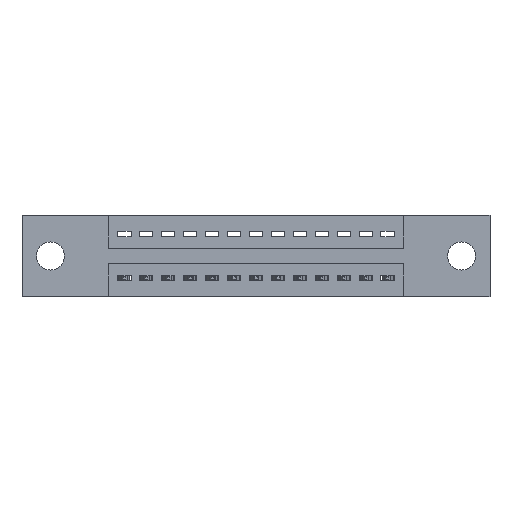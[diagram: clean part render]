
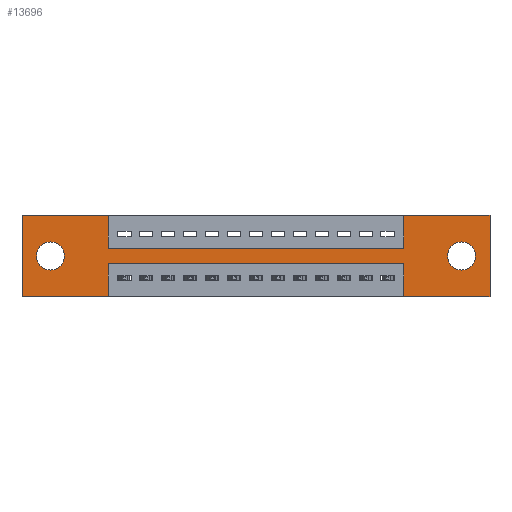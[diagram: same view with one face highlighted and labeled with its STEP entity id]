
A CAD part, front view. The second image highlights one B-rep face of the part: STEP entity #13696.
In plain terms, the highlighted planar face has unit normal (0, -1, 0).
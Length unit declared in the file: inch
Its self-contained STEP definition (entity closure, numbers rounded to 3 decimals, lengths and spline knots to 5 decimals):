
#42 = LINE ( 'NONE', #5248, #10947 ) ;
#121 = EDGE_CURVE ( 'NONE', #9580, #6579, #426, .T. ) ;
#156 = ORIENTED_EDGE ( 'NONE', *, *, #5847, .F. ) ;
#426 = LINE ( 'NONE', #842, #11322 ) ;
#506 = CIRCLE ( 'NONE', #10358, 0.064 ) ;
#594 = EDGE_CURVE ( 'NONE', #8897, #5852, #12812, .T. ) ;
#663 = EDGE_LOOP ( 'NONE', ( #5602, #11993 ) ) ;
#673 = DIRECTION ( 'NONE',  ( 1., 0., 0. ) ) ;
#752 = CARTESIAN_POINT ( 'NONE',  ( 1.7425, 0., 0. ) ) ;
#791 = DIRECTION ( 'NONE',  ( 0., 0., 1. ) ) ;
#824 = CARTESIAN_POINT ( 'NONE',  ( 0., 0., -0.37 ) ) ;
#842 = CARTESIAN_POINT ( 'NONE',  ( 1.7425, 0., 0. ) ) ;
#851 = VERTEX_POINT ( 'NONE', #7554 ) ;
#898 = CARTESIAN_POINT ( 'NONE',  ( 0.13, 0., -0.249 ) ) ;
#935 = DIRECTION ( 'NONE',  ( 0., 0., -1. ) ) ;
#994 = FACE_OUTER_BOUND ( 'NONE', #4505, .T. ) ;
#1042 = ORIENTED_EDGE ( 'NONE', *, *, #11931, .F. ) ;
#1067 = EDGE_CURVE ( 'NONE', #6768, #9808, #1173, .T. ) ;
#1142 = DIRECTION ( 'NONE',  ( 0., -1., 0. ) ) ;
#1173 = LINE ( 'NONE', #4343, #2658 ) ;
#1241 = VERTEX_POINT ( 'NONE', #6060 ) ;
#1292 = LINE ( 'NONE', #4795, #9384 ) ;
#1418 = AXIS2_PLACEMENT_3D ( 'NONE', #2308, #1142, #12689 ) ;
#1492 = CARTESIAN_POINT ( 'NONE',  ( 2.135, 0., 0. ) ) ;
#1629 = DIRECTION ( 'NONE',  ( 0., 0., -1. ) ) ;
#1669 = CARTESIAN_POINT ( 'NONE',  ( 2.005, 0., -0.185 ) ) ;
#1675 = AXIS2_PLACEMENT_3D ( 'NONE', #8307, #6896, #1629 ) ;
#2191 = ORIENTED_EDGE ( 'NONE', *, *, #8919, .F. ) ;
#2308 = CARTESIAN_POINT ( 'NONE',  ( 0., 0., -0.37 ) ) ;
#2451 = CARTESIAN_POINT ( 'NONE',  ( 0., 0., 0. ) ) ;
#2519 = DIRECTION ( 'NONE',  ( 0., 0., -1. ) ) ;
#2621 = CARTESIAN_POINT ( 'NONE',  ( 0.3925, 0., -0.22 ) ) ;
#2658 = VECTOR ( 'NONE', #12015, 39.37008 ) ;
#2685 = EDGE_LOOP ( 'NONE', ( #6090, #2816 ) ) ;
#2816 = ORIENTED_EDGE ( 'NONE', *, *, #6614, .T. ) ;
#2927 = LINE ( 'NONE', #10601, #3763 ) ;
#3255 = EDGE_CURVE ( 'NONE', #6883, #851, #2927, .T. ) ;
#3351 = LINE ( 'NONE', #7859, #8953 ) ;
#3551 = DIRECTION ( 'NONE',  ( 0., 1., 0. ) ) ;
#3587 = DIRECTION ( 'NONE',  ( 0., 0., -1. ) ) ;
#3763 = VECTOR ( 'NONE', #11692, 39.37008 ) ;
#3806 = FACE_BOUND ( 'NONE', #2685, .T. ) ;
#3917 = CARTESIAN_POINT ( 'NONE',  ( 0.3925, 0., 0. ) ) ;
#4019 = CARTESIAN_POINT ( 'NONE',  ( 0.13, 0., -0.185 ) ) ;
#4343 = CARTESIAN_POINT ( 'NONE',  ( 1.7425, 0., -0.37 ) ) ;
#4505 = EDGE_LOOP ( 'NONE', ( #13020, #1042, #9118, #7767, #9029, #156, #8680, #8380, #11028, #2191, #8775, #8261 ) ) ;
#4583 = CARTESIAN_POINT ( 'NONE',  ( 0.3925, 0., -0.37 ) ) ;
#4688 = CARTESIAN_POINT ( 'NONE',  ( 0.3925, 0., -0.15 ) ) ;
#4795 = CARTESIAN_POINT ( 'NONE',  ( 0.3925, 0., -0.15 ) ) ;
#5038 = DIRECTION ( 'NONE',  ( 0., 1., 0. ) ) ;
#5056 = CIRCLE ( 'NONE', #11271, 0.064 ) ;
#5248 = CARTESIAN_POINT ( 'NONE',  ( 0., 0., 0. ) ) ;
#5306 = PLANE ( 'NONE',  #1418 ) ;
#5480 = VECTOR ( 'NONE', #12586, 39.37008 ) ;
#5487 = VERTEX_POINT ( 'NONE', #3917 ) ;
#5600 = EDGE_CURVE ( 'NONE', #12815, #12820, #7824, .T. ) ;
#5602 = ORIENTED_EDGE ( 'NONE', *, *, #6687, .T. ) ;
#5628 = CARTESIAN_POINT ( 'NONE',  ( 0., 0., -0.37 ) ) ;
#5673 = AXIS2_PLACEMENT_3D ( 'NONE', #1669, #12535, #935 ) ;
#5828 = CARTESIAN_POINT ( 'NONE',  ( 1.7425, 0., -0.22 ) ) ;
#5830 = DIRECTION ( 'NONE',  ( -1., 0., 0. ) ) ;
#5847 = EDGE_CURVE ( 'NONE', #6579, #12815, #42, .T. ) ;
#5852 = VERTEX_POINT ( 'NONE', #12629 ) ;
#5879 = VECTOR ( 'NONE', #10864, 39.37008 ) ;
#6060 = CARTESIAN_POINT ( 'NONE',  ( 2.005, 0., -0.249 ) ) ;
#6090 = ORIENTED_EDGE ( 'NONE', *, *, #8320, .T. ) ;
#6158 = EDGE_CURVE ( 'NONE', #5852, #6883, #3351, .T. ) ;
#6435 = VERTEX_POINT ( 'NONE', #6895 ) ;
#6579 = VERTEX_POINT ( 'NONE', #752 ) ;
#6614 = EDGE_CURVE ( 'NONE', #10537, #11528, #506, .T. ) ;
#6668 = EDGE_CURVE ( 'NONE', #1241, #6435, #13417, .T. ) ;
#6687 = EDGE_CURVE ( 'NONE', #6435, #1241, #9605, .T. ) ;
#6768 = VERTEX_POINT ( 'NONE', #8556 ) ;
#6883 = VERTEX_POINT ( 'NONE', #5628 ) ;
#6895 = CARTESIAN_POINT ( 'NONE',  ( 2.005, 0., -0.121 ) ) ;
#6896 = DIRECTION ( 'NONE',  ( 0., 1., 0. ) ) ;
#7554 = CARTESIAN_POINT ( 'NONE',  ( 0., 0., 0. ) ) ;
#7653 = LINE ( 'NONE', #2451, #8467 ) ;
#7767 = ORIENTED_EDGE ( 'NONE', *, *, #8140, .F. ) ;
#7824 = LINE ( 'NONE', #1492, #9632 ) ;
#7859 = CARTESIAN_POINT ( 'NONE',  ( 0., 0., -0.37 ) ) ;
#7932 = FACE_BOUND ( 'NONE', #663, .T. ) ;
#8003 = CARTESIAN_POINT ( 'NONE',  ( 2.135, 0., 0. ) ) ;
#8091 = CARTESIAN_POINT ( 'NONE',  ( 1.7425, 0., -0.15 ) ) ;
#8140 = EDGE_CURVE ( 'NONE', #12820, #6768, #12978, .T. ) ;
#8261 = ORIENTED_EDGE ( 'NONE', *, *, #6158, .F. ) ;
#8307 = CARTESIAN_POINT ( 'NONE',  ( 2.005, 0., -0.185 ) ) ;
#8320 = EDGE_CURVE ( 'NONE', #11528, #10537, #5056, .T. ) ;
#8380 = ORIENTED_EDGE ( 'NONE', *, *, #12058, .F. ) ;
#8467 = VECTOR ( 'NONE', #10607, 39.37008 ) ;
#8556 = CARTESIAN_POINT ( 'NONE',  ( 1.7425, 0., -0.37 ) ) ;
#8593 = VERTEX_POINT ( 'NONE', #4688 ) ;
#8680 = ORIENTED_EDGE ( 'NONE', *, *, #121, .F. ) ;
#8775 = ORIENTED_EDGE ( 'NONE', *, *, #3255, .F. ) ;
#8897 = VERTEX_POINT ( 'NONE', #2621 ) ;
#8918 = CARTESIAN_POINT ( 'NONE',  ( 0.13, 0., -0.185 ) ) ;
#8919 = EDGE_CURVE ( 'NONE', #851, #5487, #7653, .T. ) ;
#8953 = VECTOR ( 'NONE', #5830, 39.37008 ) ;
#9029 = ORIENTED_EDGE ( 'NONE', *, *, #5600, .F. ) ;
#9053 = CARTESIAN_POINT ( 'NONE',  ( 2.135, 0., -0.37 ) ) ;
#9118 = ORIENTED_EDGE ( 'NONE', *, *, #1067, .F. ) ;
#9384 = VECTOR ( 'NONE', #673, 39.37008 ) ;
#9580 = VERTEX_POINT ( 'NONE', #8091 ) ;
#9605 = CIRCLE ( 'NONE', #5673, 0.064 ) ;
#9632 = VECTOR ( 'NONE', #3587, 39.37008 ) ;
#9808 = VERTEX_POINT ( 'NONE', #5828 ) ;
#10035 = VECTOR ( 'NONE', #2519, 39.37008 ) ;
#10358 = AXIS2_PLACEMENT_3D ( 'NONE', #8918, #3551, #10911 ) ;
#10537 = VERTEX_POINT ( 'NONE', #898 ) ;
#10550 = EDGE_CURVE ( 'NONE', #5487, #8593, #11083, .T. ) ;
#10601 = CARTESIAN_POINT ( 'NONE',  ( 0., 0., 0. ) ) ;
#10607 = DIRECTION ( 'NONE',  ( 1., 0., 0. ) ) ;
#10864 = DIRECTION ( 'NONE',  ( -1., 0., 0. ) ) ;
#10911 = DIRECTION ( 'NONE',  ( 0., 0., 1. ) ) ;
#10947 = VECTOR ( 'NONE', #12675, 39.37008 ) ;
#11028 = ORIENTED_EDGE ( 'NONE', *, *, #10550, .F. ) ;
#11083 = LINE ( 'NONE', #13464, #5480 ) ;
#11271 = AXIS2_PLACEMENT_3D ( 'NONE', #4019, #5038, #12133 ) ;
#11322 = VECTOR ( 'NONE', #791, 39.37008 ) ;
#11528 = VERTEX_POINT ( 'NONE', #13244 ) ;
#11678 = LINE ( 'NONE', #11950, #12853 ) ;
#11692 = DIRECTION ( 'NONE',  ( 0., 0., 1. ) ) ;
#11931 = EDGE_CURVE ( 'NONE', #9808, #8897, #11678, .T. ) ;
#11950 = CARTESIAN_POINT ( 'NONE',  ( 0.3925, 0., -0.22 ) ) ;
#11993 = ORIENTED_EDGE ( 'NONE', *, *, #6668, .T. ) ;
#12015 = DIRECTION ( 'NONE',  ( 0., 0., 1. ) ) ;
#12058 = EDGE_CURVE ( 'NONE', #8593, #9580, #1292, .T. ) ;
#12133 = DIRECTION ( 'NONE',  ( 0., 0., 1. ) ) ;
#12535 = DIRECTION ( 'NONE',  ( 0., 1., 0. ) ) ;
#12586 = DIRECTION ( 'NONE',  ( 0., 0., -1. ) ) ;
#12629 = CARTESIAN_POINT ( 'NONE',  ( 0.3925, 0., -0.37 ) ) ;
#12675 = DIRECTION ( 'NONE',  ( 1., 0., 0. ) ) ;
#12689 = DIRECTION ( 'NONE',  ( 0., 0., -1. ) ) ;
#12812 = LINE ( 'NONE', #4583, #10035 ) ;
#12815 = VERTEX_POINT ( 'NONE', #8003 ) ;
#12820 = VERTEX_POINT ( 'NONE', #9053 ) ;
#12853 = VECTOR ( 'NONE', #12917, 39.37008 ) ;
#12917 = DIRECTION ( 'NONE',  ( -1., 0., 0. ) ) ;
#12978 = LINE ( 'NONE', #824, #5879 ) ;
#13020 = ORIENTED_EDGE ( 'NONE', *, *, #594, .F. ) ;
#13244 = CARTESIAN_POINT ( 'NONE',  ( 0.13, 0., -0.121 ) ) ;
#13417 = CIRCLE ( 'NONE', #1675, 0.064 ) ;
#13464 = CARTESIAN_POINT ( 'NONE',  ( 0.3925, 0., 0. ) ) ;
#13696 = ADVANCED_FACE ( 'NONE', ( #7932, #3806, #994 ), #5306, .T. ) ;
